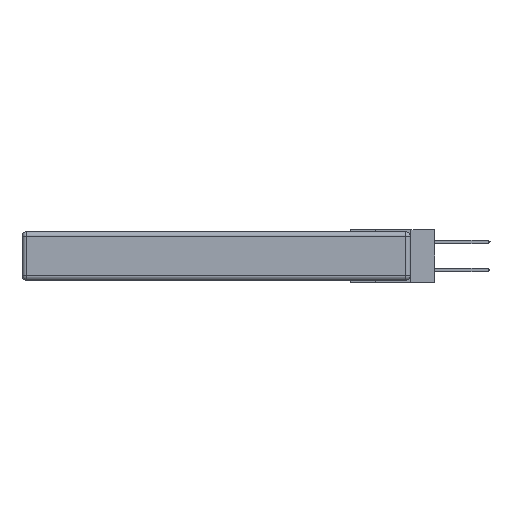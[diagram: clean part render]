
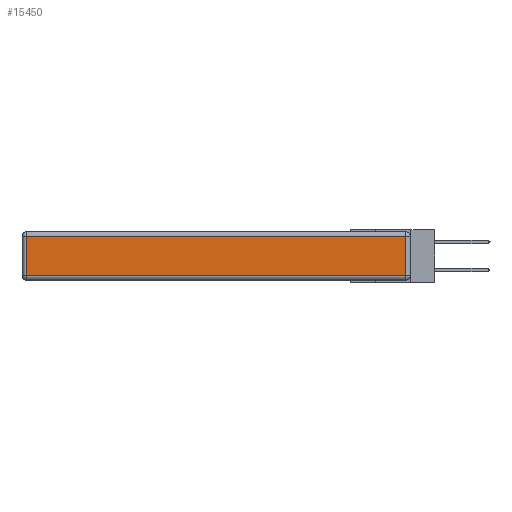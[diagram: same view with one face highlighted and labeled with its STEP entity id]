
A CAD part, left-side view. The second image highlights one B-rep face of the part: STEP entity #15450.
In plain terms, the highlighted planar face has unit normal (-1, 0, 0).
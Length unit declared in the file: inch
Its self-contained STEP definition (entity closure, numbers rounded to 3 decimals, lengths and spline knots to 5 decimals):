
#238 = DIRECTION ( 'NONE',  ( 0., 0., 1. ) ) ;
#335 = CARTESIAN_POINT ( 'NONE',  ( 0., 0.03, -0.03 ) ) ;
#929 = CARTESIAN_POINT ( 'NONE',  ( 0., 2.72, -0.343 ) ) ;
#1047 = CARTESIAN_POINT ( 'NONE',  ( 0., 2.72, -0.313 ) ) ;
#1523 = VERTEX_POINT ( 'NONE', #335 ) ;
#2272 = EDGE_CURVE ( 'NONE', #1523, #7275, #10452, .T. ) ;
#3760 = EDGE_CURVE ( 'NONE', #7275, #7093, #5598, .T. ) ;
#4074 = ORIENTED_EDGE ( 'NONE', *, *, #2272, .T. ) ;
#5023 = EDGE_CURVE ( 'NONE', #12903, #1523, #20504, .T. ) ;
#5598 = LINE ( 'NONE', #929, #17419 ) ;
#5867 = LINE ( 'NONE', #22562, #16750 ) ;
#6728 = DIRECTION ( 'NONE',  ( -1., 0., 0. ) ) ;
#7093 = VERTEX_POINT ( 'NONE', #1047 ) ;
#7178 = AXIS2_PLACEMENT_3D ( 'NONE', #11290, #6728, #13346 ) ;
#7275 = VERTEX_POINT ( 'NONE', #10131 ) ;
#8979 = CARTESIAN_POINT ( 'NONE',  ( 0., 0.03, -0.313 ) ) ;
#9644 = VECTOR ( 'NONE', #238, 39.37008 ) ;
#9781 = PLANE ( 'NONE',  #7178 ) ;
#10131 = CARTESIAN_POINT ( 'NONE',  ( 0., 2.72, -0.03 ) ) ;
#10316 = DIRECTION ( 'NONE',  ( 0., -1., 0. ) ) ;
#10452 = LINE ( 'NONE', #21804, #17790 ) ;
#10756 = DIRECTION ( 'NONE',  ( 0., 0., -1. ) ) ;
#11290 = CARTESIAN_POINT ( 'NONE',  ( 0., 0., -0.343 ) ) ;
#11531 = ORIENTED_EDGE ( 'NONE', *, *, #5023, .T. ) ;
#12903 = VERTEX_POINT ( 'NONE', #8979 ) ;
#13346 = DIRECTION ( 'NONE',  ( 0., 0., 1. ) ) ;
#15450 = ADVANCED_FACE ( 'NONE', ( #17976 ), #9781, .T. ) ;
#16750 = VECTOR ( 'NONE', #10316, 39.37008 ) ;
#17419 = VECTOR ( 'NONE', #10756, 39.37008 ) ;
#17790 = VECTOR ( 'NONE', #23919, 39.37008 ) ;
#17819 = CARTESIAN_POINT ( 'NONE',  ( 0., 0.03, -0.343 ) ) ;
#17976 = FACE_OUTER_BOUND ( 'NONE', #25192, .T. ) ;
#18561 = EDGE_CURVE ( 'NONE', #7093, #12903, #5867, .T. ) ;
#19248 = ORIENTED_EDGE ( 'NONE', *, *, #18561, .T. ) ;
#19639 = ORIENTED_EDGE ( 'NONE', *, *, #3760, .T. ) ;
#20504 = LINE ( 'NONE', #17819, #9644 ) ;
#21804 = CARTESIAN_POINT ( 'NONE',  ( 0., 2.75, -0.03 ) ) ;
#22562 = CARTESIAN_POINT ( 'NONE',  ( 0., 0., -0.313 ) ) ;
#23919 = DIRECTION ( 'NONE',  ( 0., 1., 0. ) ) ;
#25192 = EDGE_LOOP ( 'NONE', ( #19248, #11531, #4074, #19639 ) ) ;
